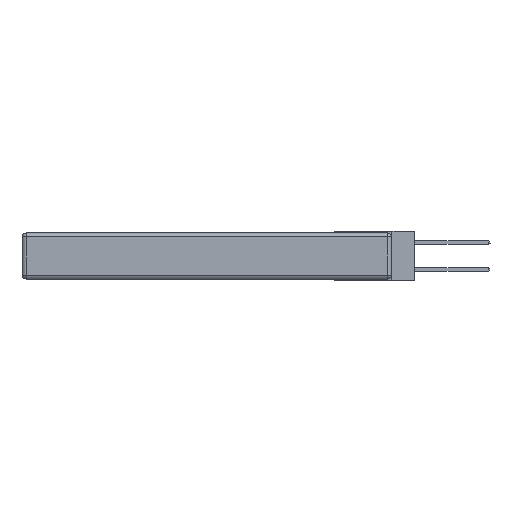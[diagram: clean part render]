
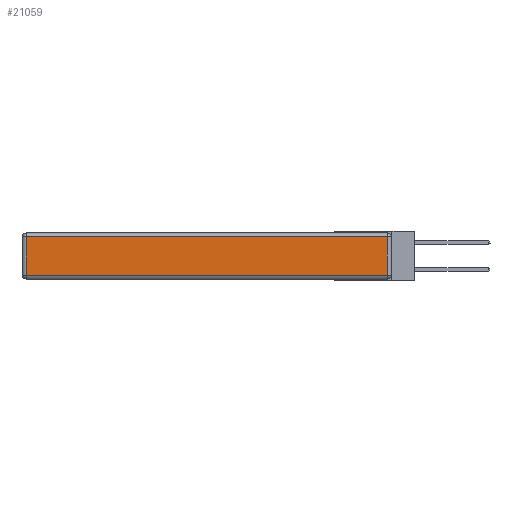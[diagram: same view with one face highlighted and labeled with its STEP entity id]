
A CAD part, left-side view. The second image highlights one B-rep face of the part: STEP entity #21059.
In plain terms, the highlighted planar face has unit normal (-1, 0, 0).
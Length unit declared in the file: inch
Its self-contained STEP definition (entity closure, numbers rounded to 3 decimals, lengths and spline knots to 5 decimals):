
#971 = LINE ( 'NONE', #10144, #21910 ) ;
#1142 = ORIENTED_EDGE ( 'NONE', *, *, #20040, .T. ) ;
#2947 = CARTESIAN_POINT ( 'NONE',  ( 0., 0., -0.313 ) ) ;
#3457 = VERTEX_POINT ( 'NONE', #24641 ) ;
#4776 = CARTESIAN_POINT ( 'NONE',  ( 0., 0., -0.343 ) ) ;
#5113 = PLANE ( 'NONE',  #22930 ) ;
#5392 = LINE ( 'NONE', #15730, #24202 ) ;
#5623 = CARTESIAN_POINT ( 'NONE',  ( 0., 2.72, -0.03 ) ) ;
#6061 = ORIENTED_EDGE ( 'NONE', *, *, #19263, .T. ) ;
#6224 = EDGE_CURVE ( 'NONE', #22125, #18782, #971, .T. ) ;
#6949 = DIRECTION ( 'NONE',  ( 0., -1., 0. ) ) ;
#7571 = LINE ( 'NONE', #18148, #8157 ) ;
#8157 = VECTOR ( 'NONE', #13943, 39.37008 ) ;
#8940 = LINE ( 'NONE', #2947, #22321 ) ;
#9764 = DIRECTION ( 'NONE',  ( 0., 0., 1. ) ) ;
#9837 = CARTESIAN_POINT ( 'NONE',  ( 0., 0.03, -0.03 ) ) ;
#10144 = CARTESIAN_POINT ( 'NONE',  ( 0., 2.75, -0.03 ) ) ;
#11186 = CARTESIAN_POINT ( 'NONE',  ( 0., 0.03, -0.313 ) ) ;
#11508 = EDGE_LOOP ( 'NONE', ( #16505, #1142, #21639, #6061 ) ) ;
#12935 = DIRECTION ( 'NONE',  ( 0., 0., 1. ) ) ;
#13575 = FACE_OUTER_BOUND ( 'NONE', #11508, .T. ) ;
#13943 = DIRECTION ( 'NONE',  ( 0., 0., -1. ) ) ;
#15351 = EDGE_CURVE ( 'NONE', #3457, #20388, #8940, .T. ) ;
#15730 = CARTESIAN_POINT ( 'NONE',  ( 0., 0.03, -0.343 ) ) ;
#16505 = ORIENTED_EDGE ( 'NONE', *, *, #15351, .T. ) ;
#18146 = DIRECTION ( 'NONE',  ( 0., 1., 0. ) ) ;
#18148 = CARTESIAN_POINT ( 'NONE',  ( 0., 2.72, -0.343 ) ) ;
#18782 = VERTEX_POINT ( 'NONE', #5623 ) ;
#19263 = EDGE_CURVE ( 'NONE', #18782, #3457, #7571, .T. ) ;
#20040 = EDGE_CURVE ( 'NONE', #20388, #22125, #5392, .T. ) ;
#20388 = VERTEX_POINT ( 'NONE', #11186 ) ;
#21059 = ADVANCED_FACE ( 'NONE', ( #13575 ), #5113, .T. ) ;
#21639 = ORIENTED_EDGE ( 'NONE', *, *, #6224, .T. ) ;
#21910 = VECTOR ( 'NONE', #18146, 39.37008 ) ;
#22125 = VERTEX_POINT ( 'NONE', #9837 ) ;
#22321 = VECTOR ( 'NONE', #6949, 39.37008 ) ;
#22333 = DIRECTION ( 'NONE',  ( -1., 0., 0. ) ) ;
#22930 = AXIS2_PLACEMENT_3D ( 'NONE', #4776, #22333, #12935 ) ;
#24202 = VECTOR ( 'NONE', #9764, 39.37008 ) ;
#24641 = CARTESIAN_POINT ( 'NONE',  ( 0., 2.72, -0.313 ) ) ;
